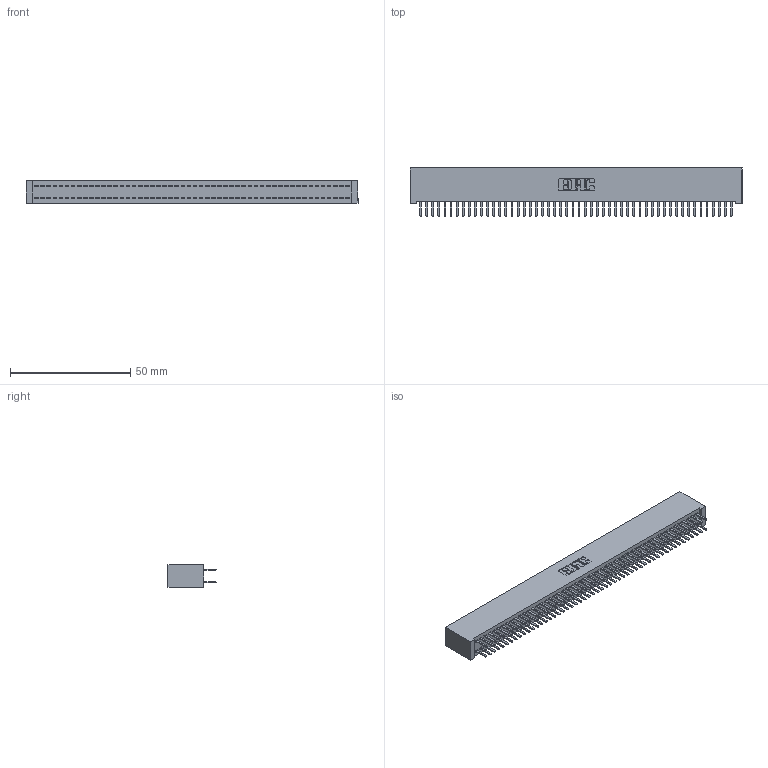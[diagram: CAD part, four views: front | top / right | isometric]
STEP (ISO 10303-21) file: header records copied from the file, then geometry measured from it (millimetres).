
FILE_DESCRIPTION (( 'STEP AP203' ), '1' );
FILE_NAME ('392-104-520-201.STEP', '2019-10-09T21:45:21', ( '' ), ( '' ), 'SwSTEP 2.0', 'SolidWorks 2016', '' );
FILE_SCHEMA (( 'CONFIG_CONTROL_DESIGN' ));
Length unit declared in the file: inch
Products named in the file (3): 342 Part_Lugless; 345-292-001_345-293-120; 392-104-520-201
Assembly tree (105 placements, depth 2):
  392-104-520-201
    342 Part_Lugless
    345-292-001_345-293-120  x104
Bounding box: 138.33 x 20.02 x 9.4 mm (x, y, z)
Volume: 12869.9 mm3; surface area: 21533.8 mm2
Topology: 105 solids, 105 shells, 5926 faces, 17227 edges, 11206 vertices
Faces by surface type: plane 4014, cylinder 1912
Entity records: 31865 total; most frequent: CARTESIAN_POINT 5278, ORIENTED_EDGE 5202, DIRECTION 4473, EDGE_CURVE 2601, LINE 2477, VECTOR 2477, VERTEX_POINT 1730, AXIS2_PLACEMENT_3D 998
